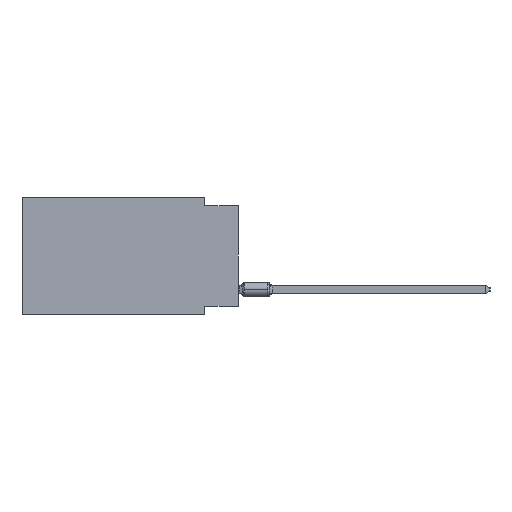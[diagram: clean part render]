
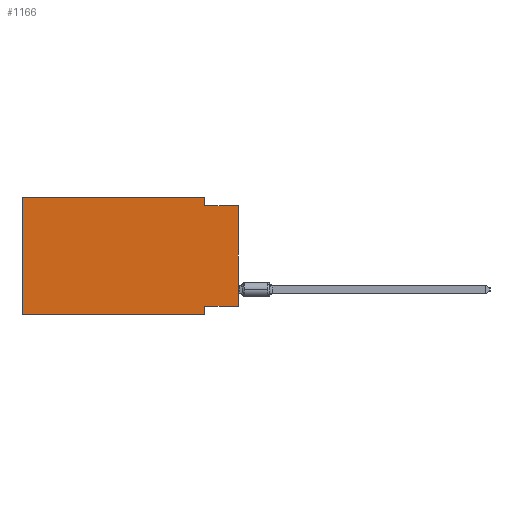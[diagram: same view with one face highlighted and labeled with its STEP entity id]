
A CAD part, left-side view. The second image highlights one B-rep face of the part: STEP entity #1166.
In plain terms, the highlighted planar face has unit normal (-1, 0, 0).
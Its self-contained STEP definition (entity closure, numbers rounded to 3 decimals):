
#613 = LINE ( 'NONE', #38376, #25036 ) ;
#997 = EDGE_CURVE ( 'NONE', #46561, #14895, #4127, .T. ) ;
#1166 = ADVANCED_FACE ( 'NONE', ( #24546 ), #47399, .F. ) ;
#1348 = LINE ( 'NONE', #45684, #16205 ) ;
#2830 = DIRECTION ( 'NONE',  ( 0., 0., -1. ) ) ;
#4082 = VECTOR ( 'NONE', #18517, 1000. ) ;
#4127 = LINE ( 'NONE', #7786, #4082 ) ;
#5838 = EDGE_CURVE ( 'NONE', #25963, #15008, #33437, .T. ) ;
#6755 = CARTESIAN_POINT ( 'NONE',  ( 0., 0., -8.255 ) ) ;
#6960 = CARTESIAN_POINT ( 'NONE',  ( 0., 2.54, -8.89 ) ) ;
#7281 = CARTESIAN_POINT ( 'NONE',  ( 0., 16.383, -8.89 ) ) ;
#7786 = CARTESIAN_POINT ( 'NONE',  ( 0., 0., 0. ) ) ;
#10417 = LINE ( 'NONE', #6755, #46018 ) ;
#11201 = DIRECTION ( 'NONE',  ( 0., 0., -1. ) ) ;
#11776 = ORIENTED_EDGE ( 'NONE', *, *, #28787, .T. ) ;
#11940 = ORIENTED_EDGE ( 'NONE', *, *, #26562, .F. ) ;
#12320 = VECTOR ( 'NONE', #11201, 1000. ) ;
#13901 = VERTEX_POINT ( 'NONE', #28679 ) ;
#14044 = DIRECTION ( 'NONE',  ( 1., 0., 0. ) ) ;
#14582 = EDGE_CURVE ( 'NONE', #13901, #43901, #47246, .T. ) ;
#14895 = VERTEX_POINT ( 'NONE', #31620 ) ;
#15008 = VERTEX_POINT ( 'NONE', #38674 ) ;
#15118 = ORIENTED_EDGE ( 'NONE', *, *, #14582, .F. ) ;
#15997 = DIRECTION ( 'NONE',  ( 0., -1., 0. ) ) ;
#16205 = VECTOR ( 'NONE', #16727, 1000. ) ;
#16727 = DIRECTION ( 'NONE',  ( 0., -1., 0. ) ) ;
#17392 = CARTESIAN_POINT ( 'NONE',  ( 0., 0., -0.635 ) ) ;
#17837 = EDGE_CURVE ( 'NONE', #15008, #47301, #1348, .T. ) ;
#18517 = DIRECTION ( 'NONE',  ( 0., 0., 1. ) ) ;
#21504 = DIRECTION ( 'NONE',  ( 0., -1., 0. ) ) ;
#22573 = LINE ( 'NONE', #30112, #35914 ) ;
#23337 = EDGE_CURVE ( 'NONE', #47301, #46330, #613, .T. ) ;
#24546 = FACE_OUTER_BOUND ( 'NONE', #39457, .T. ) ;
#25036 = VECTOR ( 'NONE', #30586, 1000. ) ;
#25260 = CARTESIAN_POINT ( 'NONE',  ( 0., 16.383, 0. ) ) ;
#25289 = DIRECTION ( 'NONE',  ( 0., 1., 0. ) ) ;
#25386 = LINE ( 'NONE', #17392, #38434 ) ;
#25963 = VERTEX_POINT ( 'NONE', #7281 ) ;
#26199 = CARTESIAN_POINT ( 'NONE',  ( 0., 2.54, -0.635 ) ) ;
#26562 = EDGE_CURVE ( 'NONE', #46330, #14895, #25386, .T. ) ;
#28679 = CARTESIAN_POINT ( 'NONE',  ( 0., 2.54, -8.255 ) ) ;
#28787 = EDGE_CURVE ( 'NONE', #25963, #43901, #22573, .T. ) ;
#28800 = ORIENTED_EDGE ( 'NONE', *, *, #31455, .F. ) ;
#29708 = CARTESIAN_POINT ( 'NONE',  ( 0., 2.54, -8.89 ) ) ;
#30112 = CARTESIAN_POINT ( 'NONE',  ( 0., 16.383, -8.89 ) ) ;
#30586 = DIRECTION ( 'NONE',  ( 0., 0., -1. ) ) ;
#30738 = CARTESIAN_POINT ( 'NONE',  ( 0., 0., -8.255 ) ) ;
#31455 = EDGE_CURVE ( 'NONE', #46561, #13901, #10417, .T. ) ;
#31620 = CARTESIAN_POINT ( 'NONE',  ( 0., 0., -0.635 ) ) ;
#32673 = ORIENTED_EDGE ( 'NONE', *, *, #17837, .F. ) ;
#33437 = LINE ( 'NONE', #37082, #34752 ) ;
#33654 = AXIS2_PLACEMENT_3D ( 'NONE', #25260, #14044, #2830 ) ;
#34752 = VECTOR ( 'NONE', #40035, 1000. ) ;
#35914 = VECTOR ( 'NONE', #15997, 1000. ) ;
#37082 = CARTESIAN_POINT ( 'NONE',  ( 0., 16.383, 0. ) ) ;
#37386 = ORIENTED_EDGE ( 'NONE', *, *, #5838, .F. ) ;
#37407 = ORIENTED_EDGE ( 'NONE', *, *, #23337, .F. ) ;
#38376 = CARTESIAN_POINT ( 'NONE',  ( 0., 2.54, 0. ) ) ;
#38434 = VECTOR ( 'NONE', #21504, 1000. ) ;
#38674 = CARTESIAN_POINT ( 'NONE',  ( 0., 16.383, 0. ) ) ;
#38675 = ORIENTED_EDGE ( 'NONE', *, *, #997, .T. ) ;
#39457 = EDGE_LOOP ( 'NONE', ( #38675, #11940, #37407, #32673, #37386, #11776, #15118, #28800 ) ) ;
#40035 = DIRECTION ( 'NONE',  ( 0., 0., 1. ) ) ;
#43901 = VERTEX_POINT ( 'NONE', #6960 ) ;
#44105 = CARTESIAN_POINT ( 'NONE',  ( 0., 2.54, 0. ) ) ;
#45684 = CARTESIAN_POINT ( 'NONE',  ( 0., 16.383, 0. ) ) ;
#46018 = VECTOR ( 'NONE', #25289, 1000. ) ;
#46330 = VERTEX_POINT ( 'NONE', #26199 ) ;
#46561 = VERTEX_POINT ( 'NONE', #30738 ) ;
#47246 = LINE ( 'NONE', #29708, #12320 ) ;
#47301 = VERTEX_POINT ( 'NONE', #44105 ) ;
#47399 = PLANE ( 'NONE',  #33654 ) ;
